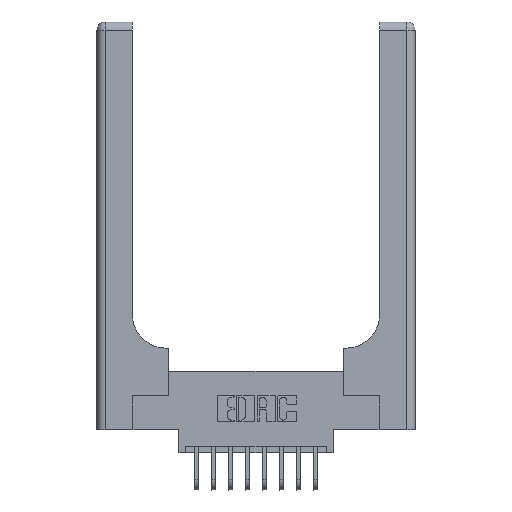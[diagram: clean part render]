
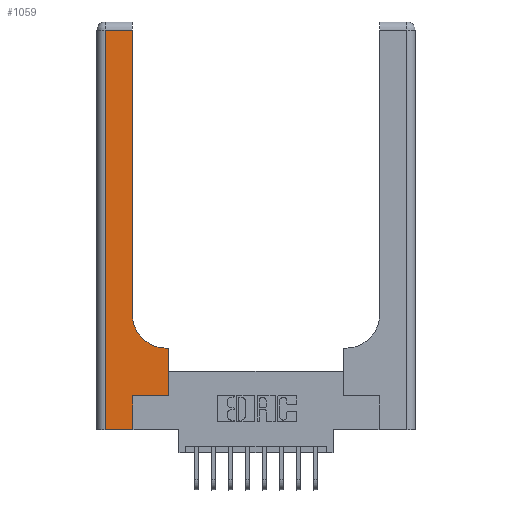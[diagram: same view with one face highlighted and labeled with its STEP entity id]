
A CAD part, top view. The second image highlights one B-rep face of the part: STEP entity #1059.
In plain terms, the highlighted planar face has unit normal (0, 0, 1).
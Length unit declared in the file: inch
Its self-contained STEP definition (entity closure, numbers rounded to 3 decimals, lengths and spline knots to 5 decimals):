
#190 = CARTESIAN_POINT ( 'NONE',  ( 0.265, 0., 0.37 ) ) ;
#291 = DIRECTION ( 'NONE',  ( -1., 0., 0. ) ) ;
#558 = EDGE_CURVE ( 'NONE', #3384, #1812, #12952, .T. ) ;
#567 = LINE ( 'NONE', #15141, #16741 ) ;
#732 = AXIS2_PLACEMENT_3D ( 'NONE', #12636, #14934, #13798 ) ;
#915 = LINE ( 'NONE', #11609, #7949 ) ;
#931 = CARTESIAN_POINT ( 'NONE',  ( 0.265, 0.25, 0.37 ) ) ;
#974 = CARTESIAN_POINT ( 'NONE',  ( 0.06, 2.94, 0.37 ) ) ;
#1059 = ADVANCED_FACE ( 'NONE', ( #2851 ), #9513, .F. ) ;
#1177 = DIRECTION ( 'NONE',  ( 1., 0., 0. ) ) ;
#1305 = LINE ( 'NONE', #14739, #10060 ) ;
#1358 = VERTEX_POINT ( 'NONE', #974 ) ;
#1744 = CARTESIAN_POINT ( 'NONE',  ( 0.265, 0.25, 0.37 ) ) ;
#1812 = VERTEX_POINT ( 'NONE', #15768 ) ;
#1894 = CARTESIAN_POINT ( 'NONE',  ( 0.265, 0., 0.37 ) ) ;
#1971 = VECTOR ( 'NONE', #3803, 39.37008 ) ;
#2595 = EDGE_CURVE ( 'NONE', #1812, #13092, #567, .T. ) ;
#2625 = VECTOR ( 'NONE', #14774, 39.37008 ) ;
#2642 = ORIENTED_EDGE ( 'NONE', *, *, #17040, .T. ) ;
#2756 = VECTOR ( 'NONE', #16718, 39.37008 ) ;
#2851 = FACE_OUTER_BOUND ( 'NONE', #13033, .T. ) ;
#3279 = EDGE_CURVE ( 'NONE', #1358, #16982, #1305, .T. ) ;
#3384 = VERTEX_POINT ( 'NONE', #1744 ) ;
#3714 = ORIENTED_EDGE ( 'NONE', *, *, #5820, .T. ) ;
#3803 = DIRECTION ( 'NONE',  ( 0., 1., 0. ) ) ;
#4150 = CARTESIAN_POINT ( 'NONE',  ( 0.26, 0.85, 0.37 ) ) ;
#5011 = CARTESIAN_POINT ( 'NONE',  ( 0.26, 2.94, 0.37 ) ) ;
#5304 = LINE ( 'NONE', #13285, #2625 ) ;
#5616 = VERTEX_POINT ( 'NONE', #190 ) ;
#5752 = ORIENTED_EDGE ( 'NONE', *, *, #2595, .T. ) ;
#5820 = EDGE_CURVE ( 'NONE', #9052, #5988, #6330, .T. ) ;
#5988 = VERTEX_POINT ( 'NONE', #4150 ) ;
#6090 = VECTOR ( 'NONE', #6766, 39.37008 ) ;
#6330 = CIRCLE ( 'NONE', #732, 0.25 ) ;
#6766 = DIRECTION ( 'NONE',  ( -1., 0., 0. ) ) ;
#6798 = CARTESIAN_POINT ( 'NONE',  ( 0., 3., 0.37 ) ) ;
#6894 = ORIENTED_EDGE ( 'NONE', *, *, #8360, .T. ) ;
#7949 = VECTOR ( 'NONE', #1177, 39.37008 ) ;
#8040 = ORIENTED_EDGE ( 'NONE', *, *, #558, .T. ) ;
#8228 = EDGE_CURVE ( 'NONE', #16982, #5616, #915, .T. ) ;
#8284 = DIRECTION ( 'NONE',  ( 0., 1., 0. ) ) ;
#8360 = EDGE_CURVE ( 'NONE', #11128, #1358, #5304, .T. ) ;
#9045 = ORIENTED_EDGE ( 'NONE', *, *, #10085, .T. ) ;
#9052 = VERTEX_POINT ( 'NONE', #12803 ) ;
#9311 = DIRECTION ( 'NONE',  ( 0., -1., 0. ) ) ;
#9425 = DIRECTION ( 'NONE',  ( 0., 0., -1. ) ) ;
#9462 = ORIENTED_EDGE ( 'NONE', *, *, #13624, .T. ) ;
#9513 = PLANE ( 'NONE',  #14861 ) ;
#10060 = VECTOR ( 'NONE', #9311, 39.37008 ) ;
#10085 = EDGE_CURVE ( 'NONE', #13092, #9052, #12001, .T. ) ;
#11128 = VERTEX_POINT ( 'NONE', #5011 ) ;
#11364 = LINE ( 'NONE', #1894, #2756 ) ;
#11609 = CARTESIAN_POINT ( 'NONE',  ( 0., 0., 0.37 ) ) ;
#11754 = VECTOR ( 'NONE', #12313, 39.37008 ) ;
#12001 = LINE ( 'NONE', #15082, #6090 ) ;
#12106 = CARTESIAN_POINT ( 'NONE',  ( 0.26, 3., 0.37 ) ) ;
#12313 = DIRECTION ( 'NONE',  ( 1., 0., 0. ) ) ;
#12334 = CARTESIAN_POINT ( 'NONE',  ( 0.528, 0.6, 0.37 ) ) ;
#12636 = CARTESIAN_POINT ( 'NONE',  ( 0.51, 0.85, 0.37 ) ) ;
#12724 = ORIENTED_EDGE ( 'NONE', *, *, #3279, .T. ) ;
#12803 = CARTESIAN_POINT ( 'NONE',  ( 0.51, 0.6, 0.37 ) ) ;
#12952 = LINE ( 'NONE', #931, #11754 ) ;
#13033 = EDGE_LOOP ( 'NONE', ( #9462, #6894, #12724, #17046, #2642, #8040, #5752, #9045, #3714 ) ) ;
#13092 = VERTEX_POINT ( 'NONE', #12334 ) ;
#13285 = CARTESIAN_POINT ( 'NONE',  ( 0., 2.94, 0.37 ) ) ;
#13579 = CARTESIAN_POINT ( 'NONE',  ( 0.06, 0., 0.37 ) ) ;
#13624 = EDGE_CURVE ( 'NONE', #5988, #11128, #17285, .T. ) ;
#13798 = DIRECTION ( 'NONE',  ( 1., 0., 0. ) ) ;
#14739 = CARTESIAN_POINT ( 'NONE',  ( 0.06, 3., 0.37 ) ) ;
#14774 = DIRECTION ( 'NONE',  ( -1., 0., 0. ) ) ;
#14861 = AXIS2_PLACEMENT_3D ( 'NONE', #6798, #9425, #291 ) ;
#14934 = DIRECTION ( 'NONE',  ( 0., 0., -1. ) ) ;
#15082 = CARTESIAN_POINT ( 'NONE',  ( 0.26, 0.6, 0.37 ) ) ;
#15141 = CARTESIAN_POINT ( 'NONE',  ( 0.528, 0.25, 0.37 ) ) ;
#15768 = CARTESIAN_POINT ( 'NONE',  ( 0.528, 0.25, 0.37 ) ) ;
#16718 = DIRECTION ( 'NONE',  ( 0., 1., 0. ) ) ;
#16741 = VECTOR ( 'NONE', #8284, 39.37008 ) ;
#16982 = VERTEX_POINT ( 'NONE', #13579 ) ;
#17040 = EDGE_CURVE ( 'NONE', #5616, #3384, #11364, .T. ) ;
#17046 = ORIENTED_EDGE ( 'NONE', *, *, #8228, .T. ) ;
#17285 = LINE ( 'NONE', #12106, #1971 ) ;
